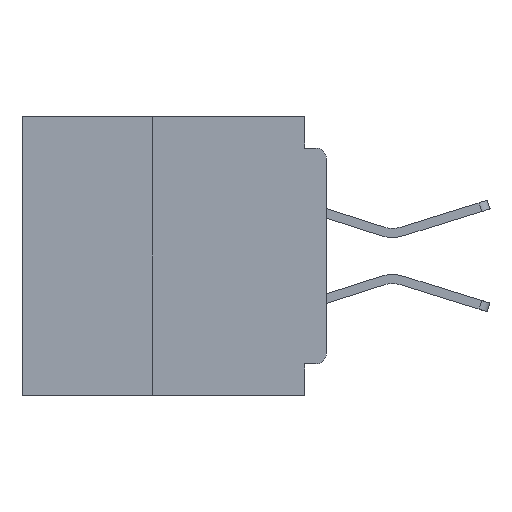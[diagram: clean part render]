
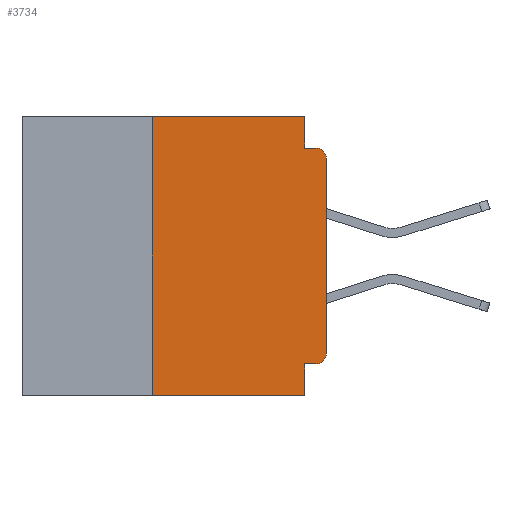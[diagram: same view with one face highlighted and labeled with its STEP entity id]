
A CAD part, left-side view. The second image highlights one B-rep face of the part: STEP entity #3734.
In plain terms, the highlighted planar face has unit normal (-1, 0, 0).
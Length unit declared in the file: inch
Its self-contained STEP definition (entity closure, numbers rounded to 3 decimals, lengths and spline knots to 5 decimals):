
#219 = LINE ( 'NONE', #27199, #40882 ) ;
#319 = DIRECTION ( 'NONE',  ( 0., -1., 0. ) ) ;
#668 = CARTESIAN_POINT ( 'NONE',  ( 0., 0.031, 0. ) ) ;
#2158 = EDGE_CURVE ( 'NONE', #9339, #8710, #45318, .T. ) ;
#3734 = ADVANCED_FACE ( 'NONE', ( #32544 ), #11798, .F. ) ;
#3891 = EDGE_CURVE ( 'NONE', #21587, #15477, #46366, .T. ) ;
#4132 = CARTESIAN_POINT ( 'NONE',  ( 0., 0.015, -0.06 ) ) ;
#4134 = ORIENTED_EDGE ( 'NONE', *, *, #22321, .F. ) ;
#6286 = CARTESIAN_POINT ( 'NONE',  ( 0., 0., -0.34 ) ) ;
#6542 = LINE ( 'NONE', #8002, #16163 ) ;
#8002 = CARTESIAN_POINT ( 'NONE',  ( 0., 0.031, -0.4 ) ) ;
#8115 = EDGE_CURVE ( 'NONE', #20596, #16187, #6542, .T. ) ;
#8243 = DIRECTION ( 'NONE',  ( 0., 0., -1. ) ) ;
#8710 = VERTEX_POINT ( 'NONE', #15862 ) ;
#8745 = EDGE_CURVE ( 'NONE', #45969, #20596, #51345, .T. ) ;
#9339 = VERTEX_POINT ( 'NONE', #19456 ) ;
#9399 = VERTEX_POINT ( 'NONE', #11581 ) ;
#10254 = ORIENTED_EDGE ( 'NONE', *, *, #3891, .F. ) ;
#10471 = EDGE_CURVE ( 'NONE', #15477, #9399, #43778, .T. ) ;
#10476 = VERTEX_POINT ( 'NONE', #38895 ) ;
#11581 = CARTESIAN_POINT ( 'NONE',  ( 0., 0.015, -0.045 ) ) ;
#11798 = PLANE ( 'NONE',  #14295 ) ;
#11816 = CARTESIAN_POINT ( 'NONE',  ( 0., 0.015, -0.355 ) ) ;
#12455 = LINE ( 'NONE', #12715, #32718 ) ;
#12715 = CARTESIAN_POINT ( 'NONE',  ( 0., 0.437, -0.4 ) ) ;
#14295 = AXIS2_PLACEMENT_3D ( 'NONE', #40102, #44162, #19995 ) ;
#14837 = CARTESIAN_POINT ( 'NONE',  ( 0., 0.031, -0.045 ) ) ;
#15477 = VERTEX_POINT ( 'NONE', #14837 ) ;
#15862 = CARTESIAN_POINT ( 'NONE',  ( 0., 0.25, 0. ) ) ;
#16163 = VECTOR ( 'NONE', #28284, 39.37008 ) ;
#16187 = VERTEX_POINT ( 'NONE', #36122 ) ;
#16791 = DIRECTION ( 'NONE',  ( 0., 0., -1. ) ) ;
#18930 = ORIENTED_EDGE ( 'NONE', *, *, #10471, .F. ) ;
#19456 = CARTESIAN_POINT ( 'NONE',  ( 0., 0.25, -0.4 ) ) ;
#19995 = DIRECTION ( 'NONE',  ( 0., 0., -1. ) ) ;
#20085 = ORIENTED_EDGE ( 'NONE', *, *, #46084, .T. ) ;
#20092 = CARTESIAN_POINT ( 'NONE',  ( 0., 0., -0.355 ) ) ;
#20596 = VERTEX_POINT ( 'NONE', #48796 ) ;
#20708 = EDGE_CURVE ( 'NONE', #45969, #38898, #45462, .T. ) ;
#21587 = VERTEX_POINT ( 'NONE', #50053 ) ;
#22321 = EDGE_CURVE ( 'NONE', #8710, #21587, #219, .T. ) ;
#23980 = DIRECTION ( 'NONE',  ( 0., 1., 0. ) ) ;
#24671 = EDGE_LOOP ( 'NONE', ( #42375, #51240, #18930, #10254, #4134, #40635, #20085, #33770, #45590, #40064 ) ) ;
#25144 = VECTOR ( 'NONE', #28848, 39.37008 ) ;
#25535 = DIRECTION ( 'NONE',  ( -1., 0., 0. ) ) ;
#26965 = AXIS2_PLACEMENT_3D ( 'NONE', #49622, #25535, #16791 ) ;
#27199 = CARTESIAN_POINT ( 'NONE',  ( 0., 0.437, 0. ) ) ;
#28120 = CIRCLE ( 'NONE', #36768, 0.015 ) ;
#28284 = DIRECTION ( 'NONE',  ( 0., 0., -1. ) ) ;
#28740 = VECTOR ( 'NONE', #23980, 39.37008 ) ;
#28848 = DIRECTION ( 'NONE',  ( 0., 0., 1. ) ) ;
#28924 = CARTESIAN_POINT ( 'NONE',  ( 0., 0.25, -0.4 ) ) ;
#29193 = DIRECTION ( 'NONE',  ( 0., 0., -1. ) ) ;
#32544 = FACE_OUTER_BOUND ( 'NONE', #24671, .T. ) ;
#32559 = DIRECTION ( 'NONE',  ( -1., 0., 0. ) ) ;
#32718 = VECTOR ( 'NONE', #319, 39.37008 ) ;
#32768 = LINE ( 'NONE', #50464, #50327 ) ;
#33042 = VECTOR ( 'NONE', #50805, 39.37008 ) ;
#33770 = ORIENTED_EDGE ( 'NONE', *, *, #8115, .F. ) ;
#34501 = DIRECTION ( 'NONE',  ( 0., 0., 1. ) ) ;
#35289 = DIRECTION ( 'NONE',  ( 0., -1., 0. ) ) ;
#35678 = VECTOR ( 'NONE', #29193, 39.37008 ) ;
#36122 = CARTESIAN_POINT ( 'NONE',  ( 0., 0.031, -0.4 ) ) ;
#36768 = AXIS2_PLACEMENT_3D ( 'NONE', #4132, #32559, #8243 ) ;
#38895 = CARTESIAN_POINT ( 'NONE',  ( 0., 0., -0.06 ) ) ;
#38898 = VERTEX_POINT ( 'NONE', #6286 ) ;
#40064 = ORIENTED_EDGE ( 'NONE', *, *, #20708, .T. ) ;
#40102 = CARTESIAN_POINT ( 'NONE',  ( 0., 0.437, 0. ) ) ;
#40635 = ORIENTED_EDGE ( 'NONE', *, *, #2158, .F. ) ;
#40882 = VECTOR ( 'NONE', #35289, 39.37008 ) ;
#42357 = EDGE_CURVE ( 'NONE', #10476, #9399, #28120, .T. ) ;
#42375 = ORIENTED_EDGE ( 'NONE', *, *, #45718, .T. ) ;
#42625 = CARTESIAN_POINT ( 'NONE',  ( 0., 0., -0.045 ) ) ;
#43778 = LINE ( 'NONE', #42625, #33042 ) ;
#44162 = DIRECTION ( 'NONE',  ( 1., 0., 0. ) ) ;
#45318 = LINE ( 'NONE', #28924, #25144 ) ;
#45462 = CIRCLE ( 'NONE', #26965, 0.015 ) ;
#45590 = ORIENTED_EDGE ( 'NONE', *, *, #8745, .F. ) ;
#45718 = EDGE_CURVE ( 'NONE', #38898, #10476, #32768, .T. ) ;
#45969 = VERTEX_POINT ( 'NONE', #11816 ) ;
#46084 = EDGE_CURVE ( 'NONE', #9339, #16187, #12455, .T. ) ;
#46366 = LINE ( 'NONE', #668, #35678 ) ;
#48796 = CARTESIAN_POINT ( 'NONE',  ( 0., 0.031, -0.355 ) ) ;
#49622 = CARTESIAN_POINT ( 'NONE',  ( 0., 0.015, -0.34 ) ) ;
#50053 = CARTESIAN_POINT ( 'NONE',  ( 0., 0.031, 0. ) ) ;
#50327 = VECTOR ( 'NONE', #34501, 39.37008 ) ;
#50464 = CARTESIAN_POINT ( 'NONE',  ( 0., 0., 0. ) ) ;
#50805 = DIRECTION ( 'NONE',  ( 0., -1., 0. ) ) ;
#51240 = ORIENTED_EDGE ( 'NONE', *, *, #42357, .T. ) ;
#51345 = LINE ( 'NONE', #20092, #28740 ) ;
